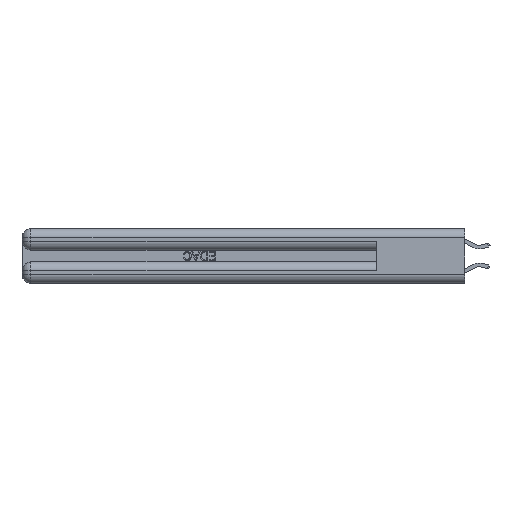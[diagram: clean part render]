
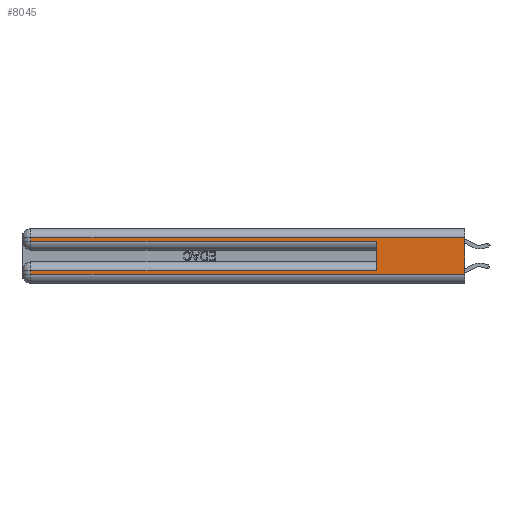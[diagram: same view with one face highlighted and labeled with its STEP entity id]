
A CAD part, left-side view. The second image highlights one B-rep face of the part: STEP entity #8045.
In plain terms, the highlighted planar face has unit normal (-1, 0, 0).
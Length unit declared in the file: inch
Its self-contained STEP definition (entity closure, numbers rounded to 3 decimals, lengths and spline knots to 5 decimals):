
#365 = CARTESIAN_POINT ( 'NONE',  ( 0., 0., 0.06 ) ) ;
#1282 = EDGE_CURVE ( 'NONE', #16009, #5902, #7271, .T. ) ;
#1971 = ORIENTED_EDGE ( 'NONE', *, *, #11234, .T. ) ;
#2229 = EDGE_LOOP ( 'NONE', ( #17573, #31490, #12751, #1971, #20411, #25997, #31072, #3498 ) ) ;
#2235 = CARTESIAN_POINT ( 'NONE',  ( 0., 0., 0.085 ) ) ;
#2605 = VECTOR ( 'NONE', #16070, 39.37008 ) ;
#3118 = EDGE_CURVE ( 'NONE', #28614, #18067, #5457, .T. ) ;
#3498 = ORIENTED_EDGE ( 'NONE', *, *, #31921, .T. ) ;
#3598 = CARTESIAN_POINT ( 'NONE',  ( 0., 0., 0.06 ) ) ;
#3896 = CARTESIAN_POINT ( 'NONE',  ( 0., 2.94, 0.06 ) ) ;
#3977 = LINE ( 'NONE', #13719, #9861 ) ;
#4188 = DIRECTION ( 'NONE',  ( 0., 0., -1. ) ) ;
#4459 = DIRECTION ( 'NONE',  ( 0., 1., 0. ) ) ;
#5457 = LINE ( 'NONE', #2235, #23222 ) ;
#5902 = VERTEX_POINT ( 'NONE', #19304 ) ;
#7271 = LINE ( 'NONE', #34648, #11863 ) ;
#8045 = ADVANCED_FACE ( 'NONE', ( #20719 ), #26872, .F. ) ;
#9606 = CARTESIAN_POINT ( 'NONE',  ( 0., 2.94, 0.37 ) ) ;
#9861 = VECTOR ( 'NONE', #13608, 39.37008 ) ;
#9970 = EDGE_CURVE ( 'NONE', #16009, #16672, #31208, .T. ) ;
#10005 = VERTEX_POINT ( 'NONE', #28282 ) ;
#11144 = DIRECTION ( 'NONE',  ( 0., -1., 0. ) ) ;
#11234 = EDGE_CURVE ( 'NONE', #10005, #29762, #17588, .T. ) ;
#11863 = VECTOR ( 'NONE', #21301, 39.37008 ) ;
#12751 = ORIENTED_EDGE ( 'NONE', *, *, #25168, .T. ) ;
#13588 = VECTOR ( 'NONE', #11144, 39.37008 ) ;
#13608 = DIRECTION ( 'NONE',  ( 0., 0., 1. ) ) ;
#13719 = CARTESIAN_POINT ( 'NONE',  ( 0., 0.6, 0.145 ) ) ;
#14384 = EDGE_CURVE ( 'NONE', #28614, #29762, #3977, .T. ) ;
#15651 = CARTESIAN_POINT ( 'NONE',  ( 0., 0., 0.37 ) ) ;
#16009 = VERTEX_POINT ( 'NONE', #23539 ) ;
#16070 = DIRECTION ( 'NONE',  ( 0., 0., -1. ) ) ;
#16108 = LINE ( 'NONE', #21139, #2605 ) ;
#16672 = VERTEX_POINT ( 'NONE', #3598 ) ;
#17172 = CARTESIAN_POINT ( 'NONE',  ( 0., 0.6, 0.285 ) ) ;
#17573 = ORIENTED_EDGE ( 'NONE', *, *, #9970, .F. ) ;
#17588 = LINE ( 'NONE', #26730, #29832 ) ;
#17671 = CARTESIAN_POINT ( 'NONE',  ( 0., 0., 0.37 ) ) ;
#17842 = LINE ( 'NONE', #365, #13588 ) ;
#18067 = VERTEX_POINT ( 'NONE', #24081 ) ;
#18387 = DIRECTION ( 'NONE',  ( 0., 0., -1. ) ) ;
#19304 = CARTESIAN_POINT ( 'NONE',  ( 0., 2.94, 0.31 ) ) ;
#20411 = ORIENTED_EDGE ( 'NONE', *, *, #14384, .F. ) ;
#20719 = FACE_OUTER_BOUND ( 'NONE', #2229, .T. ) ;
#20762 = LINE ( 'NONE', #9606, #27125 ) ;
#21049 = DIRECTION ( 'NONE',  ( 0., -1., 0. ) ) ;
#21139 = CARTESIAN_POINT ( 'NONE',  ( 0., 2.94, 0.37 ) ) ;
#21301 = DIRECTION ( 'NONE',  ( 0., 1., 0. ) ) ;
#23222 = VECTOR ( 'NONE', #4459, 39.37008 ) ;
#23539 = CARTESIAN_POINT ( 'NONE',  ( 0., 0., 0.31 ) ) ;
#23928 = DIRECTION ( 'NONE',  ( 1., 0., 0. ) ) ;
#24081 = CARTESIAN_POINT ( 'NONE',  ( 0., 2.94, 0.085 ) ) ;
#25168 = EDGE_CURVE ( 'NONE', #5902, #10005, #16108, .T. ) ;
#25997 = ORIENTED_EDGE ( 'NONE', *, *, #3118, .T. ) ;
#26235 = EDGE_CURVE ( 'NONE', #18067, #28549, #20762, .T. ) ;
#26730 = CARTESIAN_POINT ( 'NONE',  ( 0., 0., 0.285 ) ) ;
#26872 = PLANE ( 'NONE',  #31908 ) ;
#27125 = VECTOR ( 'NONE', #4188, 39.37008 ) ;
#28282 = CARTESIAN_POINT ( 'NONE',  ( 0., 2.94, 0.285 ) ) ;
#28432 = CARTESIAN_POINT ( 'NONE',  ( 0., 0.6, 0.085 ) ) ;
#28549 = VERTEX_POINT ( 'NONE', #3896 ) ;
#28614 = VERTEX_POINT ( 'NONE', #28432 ) ;
#29094 = VECTOR ( 'NONE', #31001, 39.37008 ) ;
#29762 = VERTEX_POINT ( 'NONE', #17172 ) ;
#29832 = VECTOR ( 'NONE', #21049, 39.37008 ) ;
#31001 = DIRECTION ( 'NONE',  ( 0., 0., -1. ) ) ;
#31072 = ORIENTED_EDGE ( 'NONE', *, *, #26235, .T. ) ;
#31208 = LINE ( 'NONE', #17671, #29094 ) ;
#31490 = ORIENTED_EDGE ( 'NONE', *, *, #1282, .T. ) ;
#31908 = AXIS2_PLACEMENT_3D ( 'NONE', #15651, #23928, #18387 ) ;
#31921 = EDGE_CURVE ( 'NONE', #28549, #16672, #17842, .T. ) ;
#34648 = CARTESIAN_POINT ( 'NONE',  ( 0., 0., 0.31 ) ) ;
